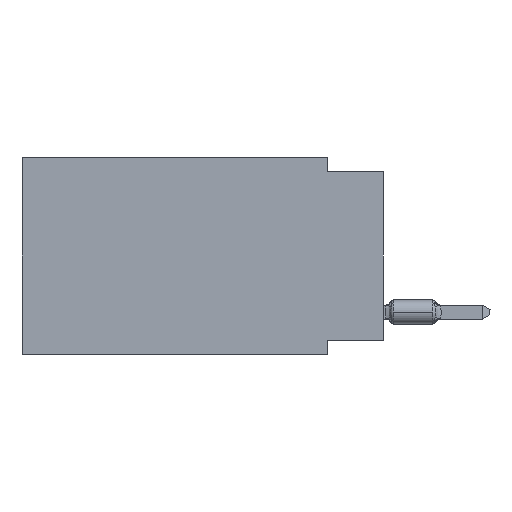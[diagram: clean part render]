
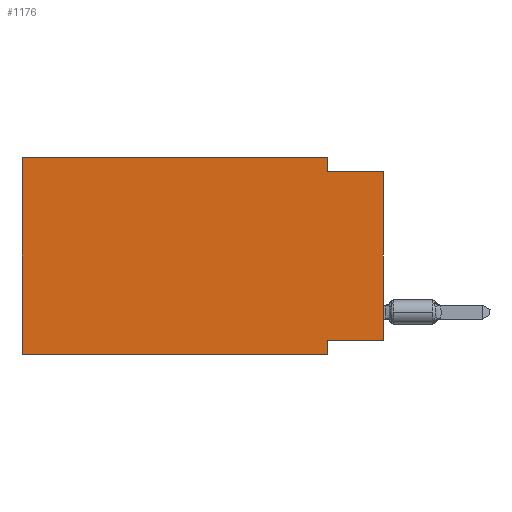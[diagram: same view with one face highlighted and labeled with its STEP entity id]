
A CAD part, left-side view. The second image highlights one B-rep face of the part: STEP entity #1176.
In plain terms, the highlighted planar face has unit normal (-1, 0, 0).
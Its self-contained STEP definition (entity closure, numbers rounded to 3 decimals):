
#53 = PLANE ( 'NONE',  #20857 ) ;
#54 = CARTESIAN_POINT ( 'NONE',  ( 0., 2.54, -8.89 ) ) ;
#1176 = ADVANCED_FACE ( 'NONE', ( #19653 ), #53, .F. ) ;
#2169 = EDGE_CURVE ( 'NONE', #36733, #26196, #40162, .T. ) ;
#3729 = CARTESIAN_POINT ( 'NONE',  ( 0., 16.383, -8.89 ) ) ;
#4582 = LINE ( 'NONE', #20635, #41274 ) ;
#5237 = CARTESIAN_POINT ( 'NONE',  ( 0., 2.54, 0. ) ) ;
#5532 = ORIENTED_EDGE ( 'NONE', *, *, #22225, .F. ) ;
#6400 = CARTESIAN_POINT ( 'NONE',  ( 0., 0., -0.635 ) ) ;
#7952 = CARTESIAN_POINT ( 'NONE',  ( 0., 0., -0.635 ) ) ;
#8808 = VERTEX_POINT ( 'NONE', #34244 ) ;
#9354 = DIRECTION ( 'NONE',  ( 0., 1., 0. ) ) ;
#10718 = DIRECTION ( 'NONE',  ( 0., 0., -1. ) ) ;
#11649 = CARTESIAN_POINT ( 'NONE',  ( 0., 2.54, -8.255 ) ) ;
#12916 = ORIENTED_EDGE ( 'NONE', *, *, #37735, .F. ) ;
#14630 = DIRECTION ( 'NONE',  ( 0., -1., 0. ) ) ;
#14943 = LINE ( 'NONE', #37072, #32211 ) ;
#15240 = VERTEX_POINT ( 'NONE', #40375 ) ;
#15919 = CARTESIAN_POINT ( 'NONE',  ( 0., 16.383, 0. ) ) ;
#16429 = CARTESIAN_POINT ( 'NONE',  ( 0., 2.54, -0.635 ) ) ;
#18956 = EDGE_CURVE ( 'NONE', #15240, #34873, #4582, .T. ) ;
#19579 = LINE ( 'NONE', #3729, #39474 ) ;
#19653 = FACE_OUTER_BOUND ( 'NONE', #34035, .T. ) ;
#20525 = VECTOR ( 'NONE', #9354, 1000. ) ;
#20635 = CARTESIAN_POINT ( 'NONE',  ( 0., 0., 0. ) ) ;
#20857 = AXIS2_PLACEMENT_3D ( 'NONE', #15919, #25730, #34933 ) ;
#22225 = EDGE_CURVE ( 'NONE', #8808, #27258, #33061, .T. ) ;
#22921 = DIRECTION ( 'NONE',  ( 0., -1., 0. ) ) ;
#23810 = LINE ( 'NONE', #7952, #26152 ) ;
#24396 = ORIENTED_EDGE ( 'NONE', *, *, #31801, .F. ) ;
#25166 = DIRECTION ( 'NONE',  ( 0., -1., 0. ) ) ;
#25639 = EDGE_CURVE ( 'NONE', #26196, #34873, #23810, .T. ) ;
#25730 = DIRECTION ( 'NONE',  ( 1., 0., 0. ) ) ;
#26152 = VECTOR ( 'NONE', #14630, 1000. ) ;
#26196 = VERTEX_POINT ( 'NONE', #16429 ) ;
#26985 = DIRECTION ( 'NONE',  ( 0., 0., 1. ) ) ;
#27258 = VERTEX_POINT ( 'NONE', #35958 ) ;
#28132 = LINE ( 'NONE', #34410, #20525 ) ;
#28451 = LINE ( 'NONE', #54, #38478 ) ;
#28458 = VERTEX_POINT ( 'NONE', #34890 ) ;
#28466 = VECTOR ( 'NONE', #26985, 1000. ) ;
#29610 = ORIENTED_EDGE ( 'NONE', *, *, #25639, .F. ) ;
#29709 = CARTESIAN_POINT ( 'NONE',  ( 0., 16.383, 0. ) ) ;
#30252 = DIRECTION ( 'NONE',  ( 0., 0., 1. ) ) ;
#31265 = EDGE_CURVE ( 'NONE', #8808, #28458, #19579, .T. ) ;
#31801 = EDGE_CURVE ( 'NONE', #15240, #32961, #28132, .T. ) ;
#32211 = VECTOR ( 'NONE', #25166, 1000. ) ;
#32961 = VERTEX_POINT ( 'NONE', #11649 ) ;
#33061 = LINE ( 'NONE', #29709, #28466 ) ;
#33182 = ORIENTED_EDGE ( 'NONE', *, *, #2169, .F. ) ;
#34035 = EDGE_LOOP ( 'NONE', ( #36882, #29610, #33182, #12916, #5532, #35380, #39903, #24396 ) ) ;
#34244 = CARTESIAN_POINT ( 'NONE',  ( 0., 16.383, -8.89 ) ) ;
#34410 = CARTESIAN_POINT ( 'NONE',  ( 0., 0., -8.255 ) ) ;
#34873 = VERTEX_POINT ( 'NONE', #6400 ) ;
#34890 = CARTESIAN_POINT ( 'NONE',  ( 0., 2.54, -8.89 ) ) ;
#34933 = DIRECTION ( 'NONE',  ( 0., 0., -1. ) ) ;
#35380 = ORIENTED_EDGE ( 'NONE', *, *, #31265, .T. ) ;
#35958 = CARTESIAN_POINT ( 'NONE',  ( 0., 16.383, 0. ) ) ;
#36317 = VECTOR ( 'NONE', #10718, 1000. ) ;
#36535 = EDGE_CURVE ( 'NONE', #32961, #28458, #28451, .T. ) ;
#36733 = VERTEX_POINT ( 'NONE', #5237 ) ;
#36882 = ORIENTED_EDGE ( 'NONE', *, *, #18956, .T. ) ;
#37072 = CARTESIAN_POINT ( 'NONE',  ( 0., 16.383, 0. ) ) ;
#37735 = EDGE_CURVE ( 'NONE', #27258, #36733, #14943, .T. ) ;
#38279 = DIRECTION ( 'NONE',  ( 0., 0., -1. ) ) ;
#38478 = VECTOR ( 'NONE', #38279, 1000. ) ;
#39338 = CARTESIAN_POINT ( 'NONE',  ( 0., 2.54, 0. ) ) ;
#39474 = VECTOR ( 'NONE', #22921, 1000. ) ;
#39903 = ORIENTED_EDGE ( 'NONE', *, *, #36535, .F. ) ;
#40162 = LINE ( 'NONE', #39338, #36317 ) ;
#40375 = CARTESIAN_POINT ( 'NONE',  ( 0., 0., -8.255 ) ) ;
#41274 = VECTOR ( 'NONE', #30252, 1000. ) ;
